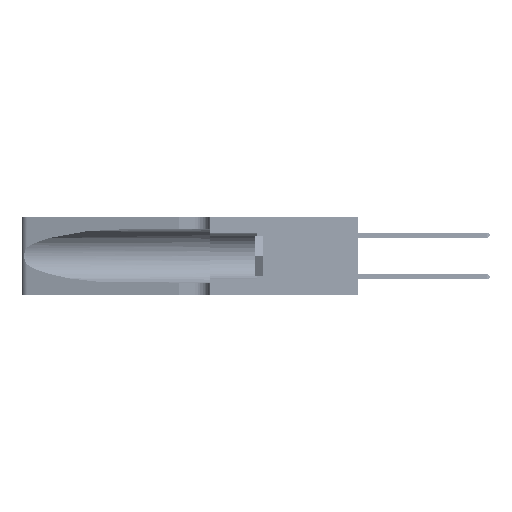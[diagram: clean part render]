
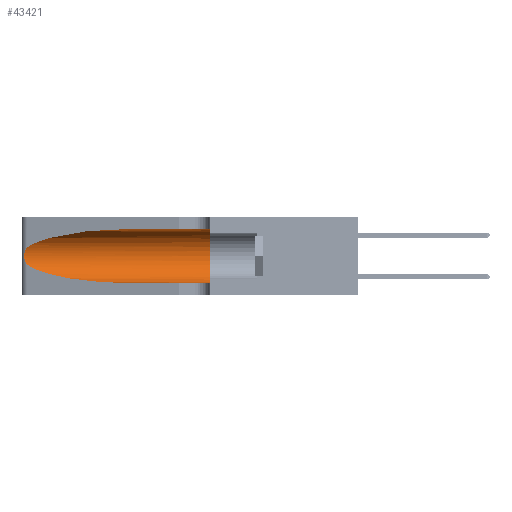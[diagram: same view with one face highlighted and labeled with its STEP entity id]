
A CAD part, left-side view. The second image highlights one B-rep face of the part: STEP entity #43421.
In plain terms, the highlighted cylindrical face has radius 3.308 mm (diameter 6.617 mm), a partial arc.
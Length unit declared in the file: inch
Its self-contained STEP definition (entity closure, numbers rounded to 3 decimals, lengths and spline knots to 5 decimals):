
#1060 = FACE_OUTER_BOUND ( 'NONE', #15965, .T. ) ;
#1287 = CARTESIAN_POINT ( 'NONE',  ( 0.25555, 1.22994, 0.2215 ) ) ;
#2043 = CARTESIAN_POINT ( 'NONE',  ( 0.18966, 0.96281, 0.31525 ) ) ;
#2326 = CARTESIAN_POINT ( 'NONE',  ( 0.1305, 0.35, 0.05475 ) ) ;
#3890 = EDGE_CURVE ( 'NONE', #20855, #28960, #18733, .T. ) ;
#5034 = AXIS2_PLACEMENT_3D ( 'NONE', #46950, #26672, #22985 ) ;
#5214 = VERTEX_POINT ( 'NONE', #28061 ) ;
#5455 = CARTESIAN_POINT ( 'NONE',  ( 0.25555, 1.22993, 0.14849 ) ) ;
#6261 = CARTESIAN_POINT ( 'NONE',  ( 0.18966, 0.96281, 0.05475 ) ) ;
#7293 = ORIENTED_EDGE ( 'NONE', *, *, #13321, .T. ) ;
#7321 = ORIENTED_EDGE ( 'NONE', *, *, #47901, .T. ) ;
#8246 = VERTEX_POINT ( 'NONE', #25479 ) ;
#9430 = CARTESIAN_POINT ( 'NONE',  ( 0.25789, 1.23486, 0.15765 ) ) ;
#9714 = CARTESIAN_POINT ( 'NONE',  ( 0.25487, 1.22718, 0.22369 ) ) ;
#9780 = ORIENTED_EDGE ( 'NONE', *, *, #47560, .F. ) ;
#10183 = DIRECTION ( 'NONE',  ( 0., 0., -1. ) ) ;
#12968 = CARTESIAN_POINT ( 'NONE',  ( 0.26075, 1.23896, 0.19203 ) ) ;
#13321 = EDGE_CURVE ( 'NONE', #8246, #5214, #26290, .T. ) ;
#13619 = CYLINDRICAL_SURFACE ( 'NONE', #44897, 0.13025 ) ;
#13762 = LINE ( 'NONE', #31742, #16187 ) ;
#14707 = CARTESIAN_POINT ( 'NONE',  ( 0.1305, 0.72297, 0.31525 ) ) ;
#14983 = VERTEX_POINT ( 'NONE', #47652 ) ;
#15965 = EDGE_LOOP ( 'NONE', ( #22119, #7293, #7321, #41865, #20036, #9780 ) ) ;
#16187 = VECTOR ( 'NONE', #16500, 39.37008 ) ;
#16500 = DIRECTION ( 'NONE',  ( 0., -1., 0. ) ) ;
#17010 = CARTESIAN_POINT ( 'NONE',  ( 0.26017, 1.23833, 0.17102 ) ) ;
#17142 = EDGE_CURVE ( 'NONE', #14983, #28960, #26875, .T. ) ;
#17928 = CARTESIAN_POINT ( 'NONE',  ( 0.25487, 1.22718, 0.14631 ) ) ;
#18733 = LINE ( 'NONE', #48748, #20605 ) ;
#18870 = DIRECTION ( 'NONE',  ( 0., -1., 0. ) ) ;
#20036 = ORIENTED_EDGE ( 'NONE', *, *, #17142, .F. ) ;
#20605 = VECTOR ( 'NONE', #18870, 39.37008 ) ;
#20845 = CARTESIAN_POINT ( 'NONE',  ( 0.25639, 1.23184, 0.21858 ) ) ;
#20855 = VERTEX_POINT ( 'NONE', #49488 ) ;
#21657 = CARTESIAN_POINT ( 'NONE',  ( 0.1305, 0.72297, 0.05475 ) ) ;
#22119 = ORIENTED_EDGE ( 'NONE', *, *, #40168, .T. ) ;
#22899 = VERTEX_POINT ( 'NONE', #46301 ) ;
#22985 = DIRECTION ( 'NONE',  ( 0., 0., 1. ) ) ;
#24800 = DIRECTION ( 'NONE',  ( 0., -1., 0. ) ) ;
#25450 = CARTESIAN_POINT ( 'NONE',  ( 0.1305, 1.61858, 0.185 ) ) ;
#25479 = CARTESIAN_POINT ( 'NONE',  ( 0.25487, 1.22718, 0.22369 ) ) ;
#26290 = B_SPLINE_CURVE_WITH_KNOTS ( 'NONE', 3,
 ( #36103, #1287, #20845, #39434, #32402, #47627, #12968, #32239, #17010, #35784, #9430, #32069, #5455, #27896 ),
 .UNSPECIFIED., .F., .F.,
 ( 4, 2, 2, 2, 2, 2, 4 ),
 ( 0., 0.00027, 0.00053, 0.00107, 0.0016, 0.00187, 0.00214 ),
 .UNSPECIFIED. ) ;
#26672 = DIRECTION ( 'NONE',  ( 0., 1., 0. ) ) ;
#26875 = CIRCLE ( 'NONE', #5034, 0.13025 ) ;
#27896 = CARTESIAN_POINT ( 'NONE',  ( 0.25487, 1.22718, 0.14631 ) ) ;
#28061 = CARTESIAN_POINT ( 'NONE',  ( 0.25487, 1.22718, 0.14631 ) ) ;
#28960 = VERTEX_POINT ( 'NONE', #2326 ) ;
#29637 = CARTESIAN_POINT ( 'NONE',  ( 0.2373, 1.15595, 0.28018 ) ) ;
#31742 = CARTESIAN_POINT ( 'NONE',  ( 0.1305, 1.61858, 0.31525 ) ) ;
#32069 = CARTESIAN_POINT ( 'NONE',  ( 0.25639, 1.23186, 0.15144 ) ) ;
#32239 = CARTESIAN_POINT ( 'NONE',  ( 0.26075, 1.23896, 0.178 ) ) ;
#32402 = CARTESIAN_POINT ( 'NONE',  ( 0.25854, 1.2359, 0.20912 ) ) ;
#35784 = CARTESIAN_POINT ( 'NONE',  ( 0.25856, 1.23593, 0.16098 ) ) ;
#36103 = CARTESIAN_POINT ( 'NONE',  ( 0.25487, 1.22718, 0.22369 ) ) ;
#36146 =( BOUNDED_CURVE ( )  B_SPLINE_CURVE ( 3, ( #17928, #37379, #6261, #21657 ),
 .UNSPECIFIED., .F., .T. ) 
 B_SPLINE_CURVE_WITH_KNOTS ( ( 4, 4 ),
 ( 3.44316, 4.71239 ),
 .UNSPECIFIED. ) 
 CURVE ( )  GEOMETRIC_REPRESENTATION_ITEM ( )  RATIONAL_B_SPLINE_CURVE ( ( 1., 0.87, 0.87, 1. ) ) 
 REPRESENTATION_ITEM ( '' )  );
#37379 = CARTESIAN_POINT ( 'NONE',  ( 0.2373, 1.15595, 0.08982 ) ) ;
#39434 = CARTESIAN_POINT ( 'NONE',  ( 0.25787, 1.23484, 0.2124 ) ) ;
#40168 = EDGE_CURVE ( 'NONE', #22899, #8246, #49306, .T. ) ;
#41865 = ORIENTED_EDGE ( 'NONE', *, *, #3890, .T. ) ;
#43421 = ADVANCED_FACE ( 'NONE', ( #1060 ), #13619, .F. ) ;
#44897 = AXIS2_PLACEMENT_3D ( 'NONE', #25450, #24800, #10183 ) ;
#46301 = CARTESIAN_POINT ( 'NONE',  ( 0.1305, 0.72297, 0.31525 ) ) ;
#46950 = CARTESIAN_POINT ( 'NONE',  ( 0.1305, 0.35, 0.185 ) ) ;
#47560 = EDGE_CURVE ( 'NONE', #22899, #14983, #13762, .T. ) ;
#47627 = CARTESIAN_POINT ( 'NONE',  ( 0.26018, 1.23835, 0.19895 ) ) ;
#47652 = CARTESIAN_POINT ( 'NONE',  ( 0.1305, 0.35, 0.31525 ) ) ;
#47901 = EDGE_CURVE ( 'NONE', #5214, #20855, #36146, .T. ) ;
#48748 = CARTESIAN_POINT ( 'NONE',  ( 0.1305, 1.61858, 0.05475 ) ) ;
#49306 =( BOUNDED_CURVE ( )  B_SPLINE_CURVE ( 3, ( #14707, #2043, #29637, #9714 ),
 .UNSPECIFIED., .F., .F. ) 
 B_SPLINE_CURVE_WITH_KNOTS ( ( 4, 4 ),
 ( 1.5708, 2.84003 ),
 .UNSPECIFIED. ) 
 CURVE ( )  GEOMETRIC_REPRESENTATION_ITEM ( )  RATIONAL_B_SPLINE_CURVE ( ( 1., 0.87, 0.87, 1. ) ) 
 REPRESENTATION_ITEM ( '' )  );
#49488 = CARTESIAN_POINT ( 'NONE',  ( 0.1305, 0.72297, 0.05475 ) ) ;
